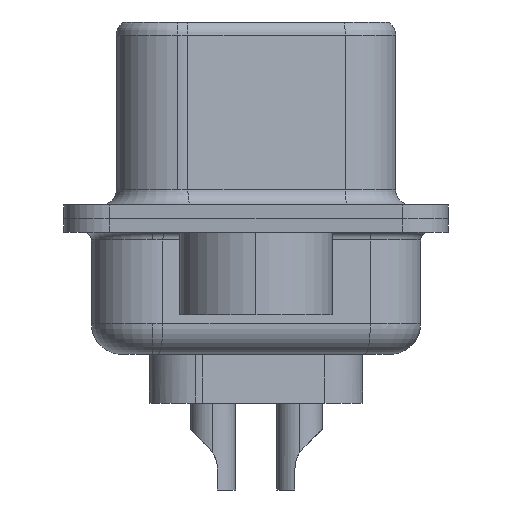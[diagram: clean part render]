
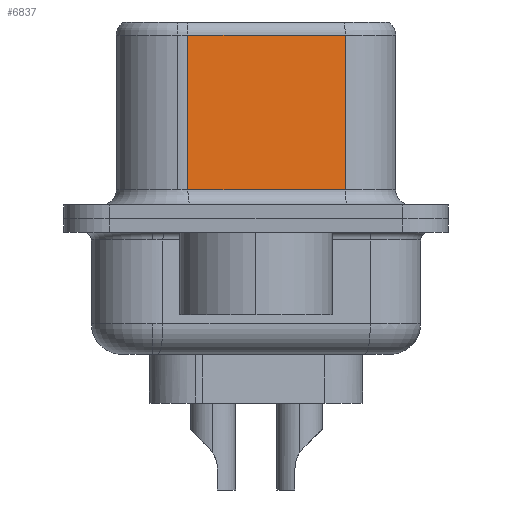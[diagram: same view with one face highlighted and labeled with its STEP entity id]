
A CAD part, left-side view. The second image highlights one B-rep face of the part: STEP entity #6837.
In plain terms, the highlighted planar face has unit normal (-0.985, -0.174, 0).
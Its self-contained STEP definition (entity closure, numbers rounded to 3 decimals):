
#1039 = VERTEX_POINT ( 'NONE', #18363 ) ;
#1278 = VERTEX_POINT ( 'NONE', #9916 ) ;
#2387 = DIRECTION ( 'NONE',  ( 0., 0., -1. ) ) ;
#3386 = EDGE_CURVE ( 'NONE', #16284, #1039, #5513, .T. ) ;
#4758 = CARTESIAN_POINT ( 'NONE',  ( 4.575, -2.927, 6.52 ) ) ;
#4821 = DIRECTION ( 'NONE',  ( 0.985, 0.174, 0. ) ) ;
#4824 = PLANE ( 'NONE',  #6703 ) ;
#5317 = CARTESIAN_POINT ( 'NONE',  ( 4.575, -2.927, 6.52 ) ) ;
#5513 = LINE ( 'NONE', #10196, #16654 ) ;
#6091 = CARTESIAN_POINT ( 'NONE',  ( 4.575, -2.927, 0.95 ) ) ;
#6386 = DIRECTION ( 'NONE',  ( -0.174, 0.985, 0. ) ) ;
#6391 = CARTESIAN_POINT ( 'NONE',  ( 3.665, 2.233, 6.02 ) ) ;
#6484 = VERTEX_POINT ( 'NONE', #18215 ) ;
#6703 = AXIS2_PLACEMENT_3D ( 'NONE', #4758, #4821, #8771 ) ;
#6837 = ADVANCED_FACE ( 'NONE', ( #16718 ), #4824, .F. ) ;
#7431 = EDGE_LOOP ( 'NONE', ( #7852, #9355, #9773, #7903 ) ) ;
#7600 = EDGE_CURVE ( 'NONE', #1278, #16284, #15420, .T. ) ;
#7852 = ORIENTED_EDGE ( 'NONE', *, *, #16431, .F. ) ;
#7903 = ORIENTED_EDGE ( 'NONE', *, *, #17355, .T. ) ;
#8771 = DIRECTION ( 'NONE',  ( -0.174, 0.985, 0. ) ) ;
#9355 = ORIENTED_EDGE ( 'NONE', *, *, #7600, .T. ) ;
#9726 = VECTOR ( 'NONE', #2387, 1000. ) ;
#9773 = ORIENTED_EDGE ( 'NONE', *, *, #3386, .T. ) ;
#9916 = CARTESIAN_POINT ( 'NONE',  ( 4.575, -2.927, 6.02 ) ) ;
#9978 = DIRECTION ( 'NONE',  ( 0., 0., -1. ) ) ;
#10196 = CARTESIAN_POINT ( 'NONE',  ( 3.665, 2.233, 6.52 ) ) ;
#10825 = VECTOR ( 'NONE', #14907, 1000. ) ;
#11436 = VECTOR ( 'NONE', #6386, 1000. ) ;
#13692 = LINE ( 'NONE', #5317, #9726 ) ;
#14872 = LINE ( 'NONE', #6091, #10825 ) ;
#14907 = DIRECTION ( 'NONE',  ( 0.174, -0.985, 0. ) ) ;
#15420 = LINE ( 'NONE', #16507, #11436 ) ;
#16284 = VERTEX_POINT ( 'NONE', #6391 ) ;
#16431 = EDGE_CURVE ( 'NONE', #1278, #6484, #13692, .T. ) ;
#16507 = CARTESIAN_POINT ( 'NONE',  ( 4.575, -2.927, 6.02 ) ) ;
#16654 = VECTOR ( 'NONE', #9978, 1000. ) ;
#16718 = FACE_OUTER_BOUND ( 'NONE', #7431, .T. ) ;
#17355 = EDGE_CURVE ( 'NONE', #1039, #6484, #14872, .T. ) ;
#18215 = CARTESIAN_POINT ( 'NONE',  ( 4.575, -2.927, 0.95 ) ) ;
#18363 = CARTESIAN_POINT ( 'NONE',  ( 3.665, 2.233, 0.95 ) ) ;
